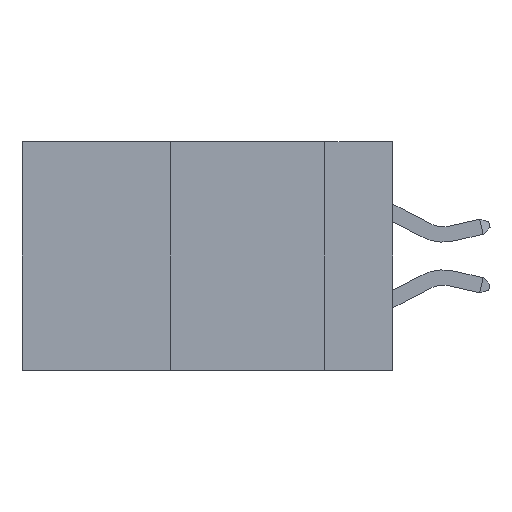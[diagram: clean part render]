
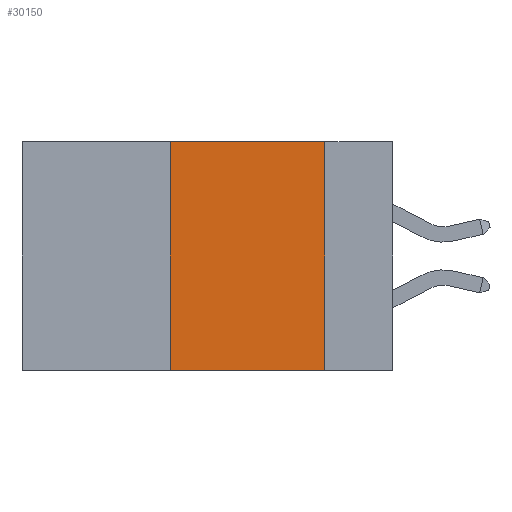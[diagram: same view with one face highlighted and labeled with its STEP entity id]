
A CAD part, left-side view. The second image highlights one B-rep face of the part: STEP entity #30150.
In plain terms, the highlighted planar face has unit normal (-1, 0, 0).
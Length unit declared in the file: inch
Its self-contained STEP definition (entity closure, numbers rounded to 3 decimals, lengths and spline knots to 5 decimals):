
#126 = LINE ( 'NONE', #21568, #15565 ) ;
#450 = ORIENTED_EDGE ( 'NONE', *, *, #27660, .F. ) ;
#754 = VECTOR ( 'NONE', #10749, 39.37008 ) ;
#2002 = EDGE_LOOP ( 'NONE', ( #450, #13351, #23793, #8645 ) ) ;
#3474 = LINE ( 'NONE', #3935, #754 ) ;
#3935 = CARTESIAN_POINT ( 'NONE',  ( 0., 0.36, 0. ) ) ;
#4484 = LINE ( 'NONE', #26251, #10068 ) ;
#5824 = FACE_OUTER_BOUND ( 'NONE', #2002, .T. ) ;
#6399 = CARTESIAN_POINT ( 'NONE',  ( 0., 0.36, 0. ) ) ;
#7986 = VERTEX_POINT ( 'NONE', #14408 ) ;
#8645 = ORIENTED_EDGE ( 'NONE', *, *, #9360, .T. ) ;
#8922 = CARTESIAN_POINT ( 'NONE',  ( 0., 0.11, -0.37 ) ) ;
#9360 = EDGE_CURVE ( 'NONE', #27398, #22326, #4484, .T. ) ;
#10068 = VECTOR ( 'NONE', #16829, 39.37008 ) ;
#10749 = DIRECTION ( 'NONE',  ( 0., 0., 1. ) ) ;
#11128 = CARTESIAN_POINT ( 'NONE',  ( 0., 0.36, -0.37 ) ) ;
#12343 = EDGE_CURVE ( 'NONE', #27398, #24080, #3474, .T. ) ;
#13351 = ORIENTED_EDGE ( 'NONE', *, *, #30415, .F. ) ;
#14408 = CARTESIAN_POINT ( 'NONE',  ( 0., 0.11, 0. ) ) ;
#15450 = DIRECTION ( 'NONE',  ( 0., 0., -1. ) ) ;
#15565 = VECTOR ( 'NONE', #23616, 39.37008 ) ;
#16829 = DIRECTION ( 'NONE',  ( 0., -1., 0. ) ) ;
#17264 = CARTESIAN_POINT ( 'NONE',  ( 0., 0.11, 0. ) ) ;
#17671 = DIRECTION ( 'NONE',  ( 1., 0., 0. ) ) ;
#20172 = CARTESIAN_POINT ( 'NONE',  ( 0., 0.6, 0. ) ) ;
#20548 = VECTOR ( 'NONE', #26846, 39.37008 ) ;
#21568 = CARTESIAN_POINT ( 'NONE',  ( 0., 0.6, 0. ) ) ;
#22326 = VERTEX_POINT ( 'NONE', #8922 ) ;
#23616 = DIRECTION ( 'NONE',  ( 0., -1., 0. ) ) ;
#23793 = ORIENTED_EDGE ( 'NONE', *, *, #12343, .F. ) ;
#24080 = VERTEX_POINT ( 'NONE', #6399 ) ;
#24114 = AXIS2_PLACEMENT_3D ( 'NONE', #20172, #17671, #15450 ) ;
#26251 = CARTESIAN_POINT ( 'NONE',  ( 0., 0.6, -0.37 ) ) ;
#26846 = DIRECTION ( 'NONE',  ( 0., 0., -1. ) ) ;
#27398 = VERTEX_POINT ( 'NONE', #11128 ) ;
#27583 = PLANE ( 'NONE',  #24114 ) ;
#27660 = EDGE_CURVE ( 'NONE', #7986, #22326, #29219, .T. ) ;
#29219 = LINE ( 'NONE', #17264, #20548 ) ;
#30150 = ADVANCED_FACE ( 'NONE', ( #5824 ), #27583, .F. ) ;
#30415 = EDGE_CURVE ( 'NONE', #24080, #7986, #126, .T. ) ;
